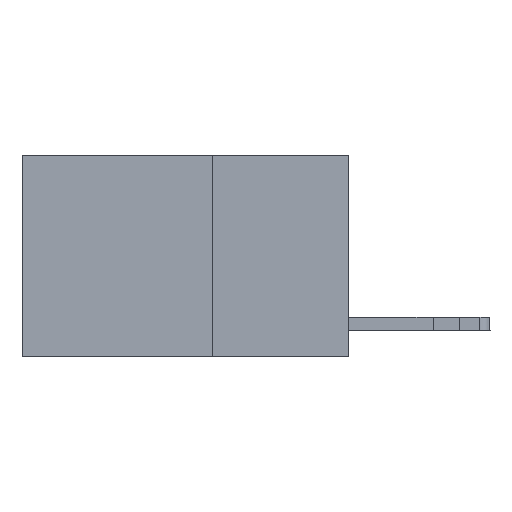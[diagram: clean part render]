
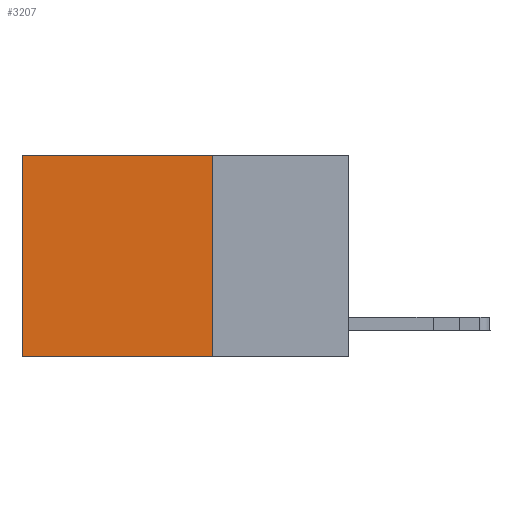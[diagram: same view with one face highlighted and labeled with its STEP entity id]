
A CAD part, left-side view. The second image highlights one B-rep face of the part: STEP entity #3207.
In plain terms, the highlighted planar face has unit normal (-1, 0, 0).
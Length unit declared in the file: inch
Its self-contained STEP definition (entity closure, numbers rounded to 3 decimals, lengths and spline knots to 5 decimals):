
#451 = VECTOR ( 'NONE', #7617, 39.37008 ) ;
#527 = PLANE ( 'NONE',  #7114 ) ;
#809 = CARTESIAN_POINT ( 'NONE',  ( 0.2625, 0.25, -0.37 ) ) ;
#810 = EDGE_CURVE ( 'NONE', #1000, #3587, #4017, .T. ) ;
#1000 = VERTEX_POINT ( 'NONE', #5804 ) ;
#1199 = CARTESIAN_POINT ( 'NONE',  ( 0.2625, 0.6, 0. ) ) ;
#1635 = VERTEX_POINT ( 'NONE', #809 ) ;
#2075 = ORIENTED_EDGE ( 'NONE', *, *, #810, .T. ) ;
#2400 = CARTESIAN_POINT ( 'NONE',  ( 0.2625, 0.25, 0. ) ) ;
#3207 = ADVANCED_FACE ( 'NONE', ( #11345 ), #527, .F. ) ;
#3324 = LINE ( 'NONE', #12682, #451 ) ;
#3535 = VERTEX_POINT ( 'NONE', #6109 ) ;
#3587 = VERTEX_POINT ( 'NONE', #1199 ) ;
#4017 = LINE ( 'NONE', #11291, #11925 ) ;
#4932 = ORIENTED_EDGE ( 'NONE', *, *, #7266, .T. ) ;
#5011 = EDGE_LOOP ( 'NONE', ( #4932, #6251, #10200, #2075 ) ) ;
#5804 = CARTESIAN_POINT ( 'NONE',  ( 0.2625, 0.25, 0. ) ) ;
#6069 = LINE ( 'NONE', #10550, #11244 ) ;
#6109 = CARTESIAN_POINT ( 'NONE',  ( 0.2625, 0.6, -0.37 ) ) ;
#6251 = ORIENTED_EDGE ( 'NONE', *, *, #8485, .F. ) ;
#7114 = AXIS2_PLACEMENT_3D ( 'NONE', #11720, #10682, #9903 ) ;
#7243 = EDGE_CURVE ( 'NONE', #1000, #1635, #8802, .T. ) ;
#7266 = EDGE_CURVE ( 'NONE', #3587, #3535, #3324, .T. ) ;
#7575 = DIRECTION ( 'NONE',  ( 0., 0., -1. ) ) ;
#7617 = DIRECTION ( 'NONE',  ( 0., 0., -1. ) ) ;
#8485 = EDGE_CURVE ( 'NONE', #1635, #3535, #6069, .T. ) ;
#8495 = DIRECTION ( 'NONE',  ( 0., 1., 0. ) ) ;
#8802 = LINE ( 'NONE', #2400, #11617 ) ;
#9903 = DIRECTION ( 'NONE',  ( 0., 0., -1. ) ) ;
#10200 = ORIENTED_EDGE ( 'NONE', *, *, #7243, .F. ) ;
#10550 = CARTESIAN_POINT ( 'NONE',  ( 0.2625, 0.25, -0.37 ) ) ;
#10682 = DIRECTION ( 'NONE',  ( 1., 0., 0. ) ) ;
#11244 = VECTOR ( 'NONE', #8495, 39.37008 ) ;
#11291 = CARTESIAN_POINT ( 'NONE',  ( 0.2625, 0.25, 0. ) ) ;
#11345 = FACE_OUTER_BOUND ( 'NONE', #5011, .T. ) ;
#11617 = VECTOR ( 'NONE', #7575, 39.37008 ) ;
#11720 = CARTESIAN_POINT ( 'NONE',  ( 0.2625, 0.25, 0. ) ) ;
#11925 = VECTOR ( 'NONE', #12346, 39.37008 ) ;
#12346 = DIRECTION ( 'NONE',  ( 0., 1., 0. ) ) ;
#12682 = CARTESIAN_POINT ( 'NONE',  ( 0.2625, 0.6, 0. ) ) ;
